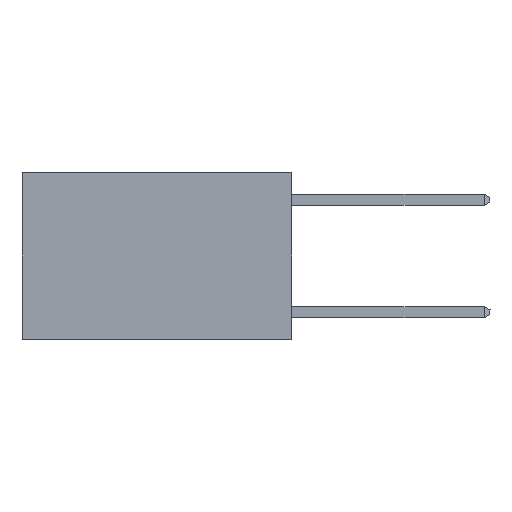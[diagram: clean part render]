
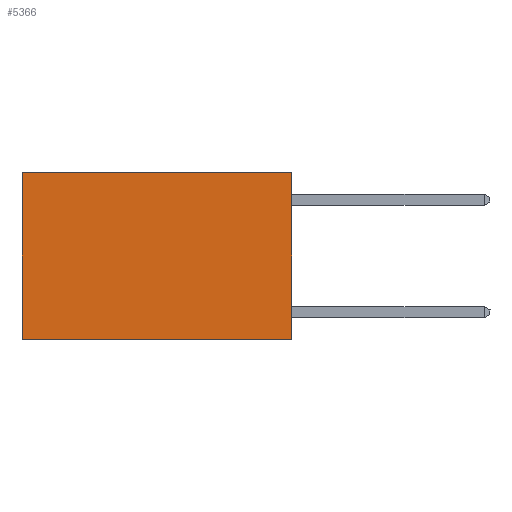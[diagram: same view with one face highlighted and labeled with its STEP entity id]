
A CAD part, left-side view. The second image highlights one B-rep face of the part: STEP entity #5366.
In plain terms, the highlighted planar face has unit normal (-1, 0, 0).
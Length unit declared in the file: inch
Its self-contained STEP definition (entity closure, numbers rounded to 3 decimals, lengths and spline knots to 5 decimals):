
#821 = VERTEX_POINT ( 'NONE', #1913 ) ;
#1205 = FACE_OUTER_BOUND ( 'NONE', #6324, .T. ) ;
#1255 = CARTESIAN_POINT ( 'NONE',  ( 0.2625, 0., 0. ) ) ;
#1289 = DIRECTION ( 'NONE',  ( 0., 1., 0. ) ) ;
#1813 = LINE ( 'NONE', #8155, #6249 ) ;
#1913 = CARTESIAN_POINT ( 'NONE',  ( 0.2625, 0., 0. ) ) ;
#2066 = CARTESIAN_POINT ( 'NONE',  ( 0.2625, 0.6, -0.37 ) ) ;
#2161 = VECTOR ( 'NONE', #1289, 39.37008 ) ;
#2215 = VERTEX_POINT ( 'NONE', #5980 ) ;
#2247 = DIRECTION ( 'NONE',  ( 0., 0., -1. ) ) ;
#3090 = AXIS2_PLACEMENT_3D ( 'NONE', #1255, #7409, #2247 ) ;
#3432 = ORIENTED_EDGE ( 'NONE', *, *, #9233, .T. ) ;
#3524 = ORIENTED_EDGE ( 'NONE', *, *, #5316, .F. ) ;
#3563 = ORIENTED_EDGE ( 'NONE', *, *, #9528, .F. ) ;
#3573 = ORIENTED_EDGE ( 'NONE', *, *, #9515, .T. ) ;
#4081 = CARTESIAN_POINT ( 'NONE',  ( 0.2625, 0., 0. ) ) ;
#4532 = LINE ( 'NONE', #4927, #2161 ) ;
#4805 = VECTOR ( 'NONE', #9055, 39.37008 ) ;
#4927 = CARTESIAN_POINT ( 'NONE',  ( 0.2625, 0., 0. ) ) ;
#5316 = EDGE_CURVE ( 'NONE', #7094, #10031, #1813, .T. ) ;
#5366 = ADVANCED_FACE ( 'NONE', ( #1205 ), #6569, .F. ) ;
#5504 = VECTOR ( 'NONE', #6259, 39.37008 ) ;
#5980 = CARTESIAN_POINT ( 'NONE',  ( 0.2625, 0.6, 0. ) ) ;
#6198 = CARTESIAN_POINT ( 'NONE',  ( 0.2625, 0.6, 0. ) ) ;
#6249 = VECTOR ( 'NONE', #9726, 39.37008 ) ;
#6259 = DIRECTION ( 'NONE',  ( 0., 0., -1. ) ) ;
#6303 = CARTESIAN_POINT ( 'NONE',  ( 0.2625, 0., -0.37 ) ) ;
#6324 = EDGE_LOOP ( 'NONE', ( #3432, #3524, #3563, #3573 ) ) ;
#6569 = PLANE ( 'NONE',  #3090 ) ;
#7094 = VERTEX_POINT ( 'NONE', #6303 ) ;
#7409 = DIRECTION ( 'NONE',  ( 1., 0., 0. ) ) ;
#8155 = CARTESIAN_POINT ( 'NONE',  ( 0.2625, 0., -0.37 ) ) ;
#9055 = DIRECTION ( 'NONE',  ( 0., 0., -1. ) ) ;
#9233 = EDGE_CURVE ( 'NONE', #2215, #10031, #9814, .T. ) ;
#9515 = EDGE_CURVE ( 'NONE', #821, #2215, #4532, .T. ) ;
#9528 = EDGE_CURVE ( 'NONE', #821, #7094, #10815, .T. ) ;
#9726 = DIRECTION ( 'NONE',  ( 0., 1., 0. ) ) ;
#9814 = LINE ( 'NONE', #6198, #5504 ) ;
#10031 = VERTEX_POINT ( 'NONE', #2066 ) ;
#10815 = LINE ( 'NONE', #4081, #4805 ) ;
